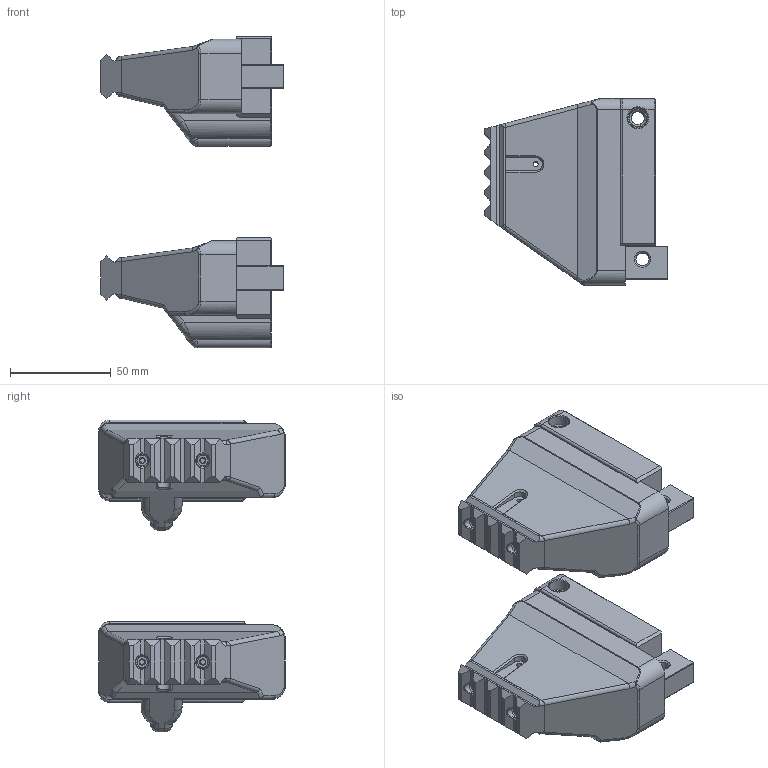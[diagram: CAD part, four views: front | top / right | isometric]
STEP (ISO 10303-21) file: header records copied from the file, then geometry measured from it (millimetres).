
FILE_DESCRIPTION(/* description */ (''),/* implementation_level */ '2;1');
FILE_NAME(/* name */ 'mod9 v2 and v3 extended endcaps.stp',/* time_stamp */ '2021-01-24T23:10:39+02:00',/* author */ (''),/* organization */ (''),/* preprocessor_version */ 'ST-DEVELOPER v15.2',/* originating_system */ 'Autodesk Translator Framework v2.0.0.5431',/* authorisation */ '');
FILE_SCHEMA (('AUTOMOTIVE_DESIGN { 1 0 10303 214 3 1 1 }'));
Length unit declared in the file: centimetre
Products named in the file (1): mod9 v2 v3 fixed endcap d
Bounding box: 90.62 x 92.64 x 154.82 mm (x, y, z)
Volume: 351573.1 mm3; surface area: 70866.2 mm2
Topology: 4 solids, 4 shells, 569 faces, 1439 edges, 886 vertices
Faces by surface type: plane 284, cylinder 142, bspline 67, cone 40, torus 24, sphere 12
Full cylindrical faces by diameter (mm): 2.5 x8, 3.1 x4, 4 x2, 6.5 x10, 10 x4, 13 x2, 20.4 x2, 23.4 x2, 27.4 x2
Entity records: 19903 total; most frequent: CARTESIAN_POINT 6844, ORIENTED_EDGE 2706, DIRECTION 2567, EDGE_CURVE 1353, AXIS2_PLACEMENT_3D 871, VERTEX_POINT 868, LINE 825, VECTOR 825
